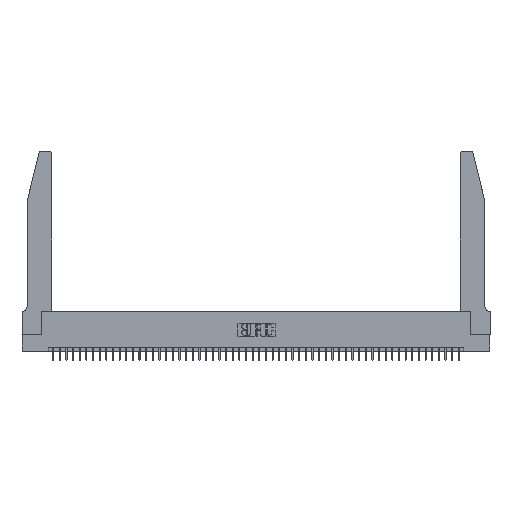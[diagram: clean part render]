
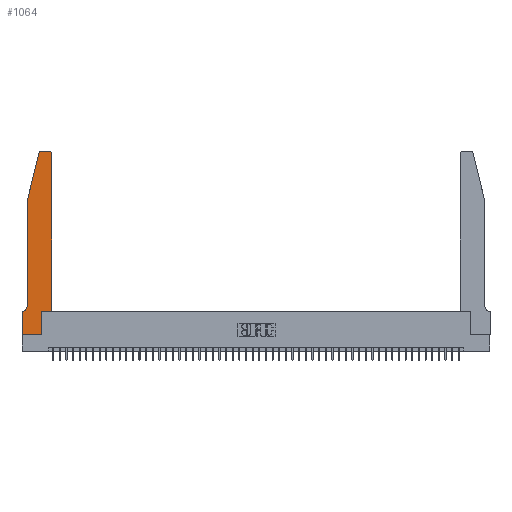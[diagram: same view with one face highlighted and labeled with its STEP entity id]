
A CAD part, top view. The second image highlights one B-rep face of the part: STEP entity #1064.
In plain terms, the highlighted planar face has unit normal (0, 0, 1).
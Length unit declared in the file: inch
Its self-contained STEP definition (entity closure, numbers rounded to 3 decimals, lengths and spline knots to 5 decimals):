
#1064 = ADVANCED_FACE ( 'NONE', ( #33381 ), #32877, .T. ) ;
#2428 = EDGE_CURVE ( 'NONE', #46114, #42093, #40867, .T. ) ;
#2537 = EDGE_CURVE ( 'NONE', #34279, #43101, #37245, .T. ) ;
#2688 = CARTESIAN_POINT ( 'NONE',  ( 0., 0.35, 0.37 ) ) ;
#3288 = EDGE_CURVE ( 'NONE', #28973, #42106, #38147, .T. ) ;
#3740 = CARTESIAN_POINT ( 'NONE',  ( 0.2865, 0.35, 0.37 ) ) ;
#4291 = DIRECTION ( 'NONE',  ( 0., 0., 1. ) ) ;
#5015 = ORIENTED_EDGE ( 'NONE', *, *, #2537, .T. ) ;
#5049 = EDGE_CURVE ( 'NONE', #45763, #29355, #19992, .T. ) ;
#5088 = EDGE_CURVE ( 'NONE', #43101, #45763, #33929, .T. ) ;
#5611 = DIRECTION ( 'NONE',  ( -0.239, -0.971, 0. ) ) ;
#6374 = CARTESIAN_POINT ( 'NONE',  ( 0.4505, 0.35, 0.37 ) ) ;
#6752 = DIRECTION ( 'NONE',  ( 0., -1., 0. ) ) ;
#6981 = ORIENTED_EDGE ( 'NONE', *, *, #20315, .T. ) ;
#7012 = EDGE_CURVE ( 'NONE', #25494, #46114, #38992, .T. ) ;
#7076 = VERTEX_POINT ( 'NONE', #47707 ) ;
#7949 = CARTESIAN_POINT ( 'NONE',  ( 0.2865, 0.35, 0.37 ) ) ;
#8156 = LINE ( 'NONE', #16876, #20781 ) ;
#8288 = CARTESIAN_POINT ( 'NONE',  ( 0., 0., 0.37 ) ) ;
#8512 = LINE ( 'NONE', #36561, #22641 ) ;
#9117 = EDGE_CURVE ( 'NONE', #7076, #31902, #8512, .T. ) ;
#10835 = EDGE_LOOP ( 'NONE', ( #27626, #48639, #5015, #48034, #19492, #50572, #36149, #48231, #27034, #12563, #15270, #6981 ) ) ;
#11170 = CARTESIAN_POINT ( 'NONE',  ( 0.0755, 0.42, 0.37 ) ) ;
#11442 = EDGE_CURVE ( 'NONE', #31902, #34279, #32634, .T. ) ;
#12353 = EDGE_CURVE ( 'NONE', #42106, #25494, #43546, .T. ) ;
#12563 = ORIENTED_EDGE ( 'NONE', *, *, #2428, .T. ) ;
#13418 = AXIS2_PLACEMENT_3D ( 'NONE', #49366, #30817, #19238 ) ;
#13761 = LINE ( 'NONE', #14017, #16633 ) ;
#14017 = CARTESIAN_POINT ( 'NONE',  ( 0.0755, 0.35, 0.37 ) ) ;
#15270 = ORIENTED_EDGE ( 'NONE', *, *, #24797, .T. ) ;
#15335 = CARTESIAN_POINT ( 'NONE',  ( 0., 0., 0.37 ) ) ;
#16633 = VECTOR ( 'NONE', #29454, 39.37008 ) ;
#16876 = CARTESIAN_POINT ( 'NONE',  ( 0.4505, 0.35, 0.37 ) ) ;
#17863 = VERTEX_POINT ( 'NONE', #49864 ) ;
#17963 = DIRECTION ( 'NONE',  ( 1., 0., 0. ) ) ;
#19011 = AXIS2_PLACEMENT_3D ( 'NONE', #36835, #33741, #29093 ) ;
#19238 = DIRECTION ( 'NONE',  ( -1., 0., 0. ) ) ;
#19441 = DIRECTION ( 'NONE',  ( 0., 1., 0. ) ) ;
#19492 = ORIENTED_EDGE ( 'NONE', *, *, #5049, .T. ) ;
#19992 = CIRCLE ( 'NONE', #13418, 0.07 ) ;
#20100 = VECTOR ( 'NONE', #19441, 39.37008 ) ;
#20315 = EDGE_CURVE ( 'NONE', #17863, #7076, #20605, .T. ) ;
#20605 = CIRCLE ( 'NONE', #19011, 0.03 ) ;
#20781 = VECTOR ( 'NONE', #39790, 39.37008 ) ;
#22641 = VECTOR ( 'NONE', #36827, 39.37008 ) ;
#23843 = CARTESIAN_POINT ( 'NONE',  ( 0.284, 2.72, 0.37 ) ) ;
#24797 = EDGE_CURVE ( 'NONE', #42093, #17863, #8156, .T. ) ;
#25494 = VERTEX_POINT ( 'NONE', #26983 ) ;
#26983 = CARTESIAN_POINT ( 'NONE',  ( 0.2865, 0., 0.37 ) ) ;
#27034 = ORIENTED_EDGE ( 'NONE', *, *, #7012, .T. ) ;
#27626 = ORIENTED_EDGE ( 'NONE', *, *, #9117, .T. ) ;
#28496 = CARTESIAN_POINT ( 'NONE',  ( 0., 0.35, 0.37 ) ) ;
#28973 = VERTEX_POINT ( 'NONE', #2688 ) ;
#29093 = DIRECTION ( 'NONE',  ( 1., 0., 0. ) ) ;
#29355 = VERTEX_POINT ( 'NONE', #37905 ) ;
#29454 = DIRECTION ( 'NONE',  ( -1., 0., 0. ) ) ;
#30817 = DIRECTION ( 'NONE',  ( 0., 0., -1. ) ) ;
#31902 = VERTEX_POINT ( 'NONE', #49010 ) ;
#32516 = VECTOR ( 'NONE', #17963, 39.37008 ) ;
#32634 = CIRCLE ( 'NONE', #44978, 0.03 ) ;
#32877 = PLANE ( 'NONE',  #43920 ) ;
#33381 = FACE_OUTER_BOUND ( 'NONE', #10835, .T. ) ;
#33741 = DIRECTION ( 'NONE',  ( 0., 0., 1. ) ) ;
#33929 = LINE ( 'NONE', #42673, #41396 ) ;
#34279 = VERTEX_POINT ( 'NONE', #47973 ) ;
#35271 = CARTESIAN_POINT ( 'NONE',  ( 0.0755, 2., 0.37 ) ) ;
#35336 = VECTOR ( 'NONE', #5611, 39.37008 ) ;
#36149 = ORIENTED_EDGE ( 'NONE', *, *, #3288, .T. ) ;
#36561 = CARTESIAN_POINT ( 'NONE',  ( 0.2605, 2.75, 0.37 ) ) ;
#36739 = DIRECTION ( 'NONE',  ( 1., 0., 0. ) ) ;
#36827 = DIRECTION ( 'NONE',  ( -1., 0., 0. ) ) ;
#36835 = CARTESIAN_POINT ( 'NONE',  ( 0.4205, 2.72, 0.37 ) ) ;
#37035 = CARTESIAN_POINT ( 'NONE',  ( 0.4505, 0.35, 0.37 ) ) ;
#37245 = LINE ( 'NONE', #41122, #35336 ) ;
#37643 = VECTOR ( 'NONE', #39933, 39.37008 ) ;
#37905 = CARTESIAN_POINT ( 'NONE',  ( 0.0055, 0.35, 0.37 ) ) ;
#38147 = LINE ( 'NONE', #50233, #39609 ) ;
#38992 = LINE ( 'NONE', #3740, #20100 ) ;
#39609 = VECTOR ( 'NONE', #6752, 39.37008 ) ;
#39790 = DIRECTION ( 'NONE',  ( 0., 1., 0. ) ) ;
#39933 = DIRECTION ( 'NONE',  ( 1., 0., 0. ) ) ;
#40330 = DIRECTION ( 'NONE',  ( 0., 0., 1. ) ) ;
#40867 = LINE ( 'NONE', #6374, #32516 ) ;
#41122 = CARTESIAN_POINT ( 'NONE',  ( 0.0755, 2., 0.37 ) ) ;
#41396 = VECTOR ( 'NONE', #50371, 39.37008 ) ;
#42093 = VERTEX_POINT ( 'NONE', #37035 ) ;
#42106 = VERTEX_POINT ( 'NONE', #15335 ) ;
#42673 = CARTESIAN_POINT ( 'NONE',  ( 0.0755, 2., 0.37 ) ) ;
#43101 = VERTEX_POINT ( 'NONE', #35271 ) ;
#43546 = LINE ( 'NONE', #8288, #37643 ) ;
#43920 = AXIS2_PLACEMENT_3D ( 'NONE', #28496, #40330, #36739 ) ;
#44978 = AXIS2_PLACEMENT_3D ( 'NONE', #23843, #4291, #47765 ) ;
#45594 = EDGE_CURVE ( 'NONE', #29355, #28973, #13761, .T. ) ;
#45763 = VERTEX_POINT ( 'NONE', #11170 ) ;
#46114 = VERTEX_POINT ( 'NONE', #7949 ) ;
#47707 = CARTESIAN_POINT ( 'NONE',  ( 0.4205, 2.75, 0.37 ) ) ;
#47765 = DIRECTION ( 'NONE',  ( 1., 0., 0. ) ) ;
#47973 = CARTESIAN_POINT ( 'NONE',  ( 0.25487, 2.72718, 0.37 ) ) ;
#48034 = ORIENTED_EDGE ( 'NONE', *, *, #5088, .T. ) ;
#48231 = ORIENTED_EDGE ( 'NONE', *, *, #12353, .T. ) ;
#48639 = ORIENTED_EDGE ( 'NONE', *, *, #11442, .T. ) ;
#49010 = CARTESIAN_POINT ( 'NONE',  ( 0.284, 2.75, 0.37 ) ) ;
#49366 = CARTESIAN_POINT ( 'NONE',  ( 0.0055, 0.42, 0.37 ) ) ;
#49864 = CARTESIAN_POINT ( 'NONE',  ( 0.4505, 2.72, 0.37 ) ) ;
#50233 = CARTESIAN_POINT ( 'NONE',  ( 0., 0., 0.37 ) ) ;
#50371 = DIRECTION ( 'NONE',  ( 0., -1., 0. ) ) ;
#50572 = ORIENTED_EDGE ( 'NONE', *, *, #45594, .T. ) ;
